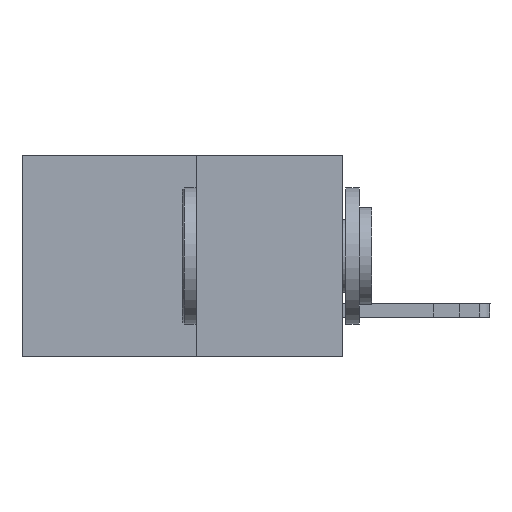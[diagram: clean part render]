
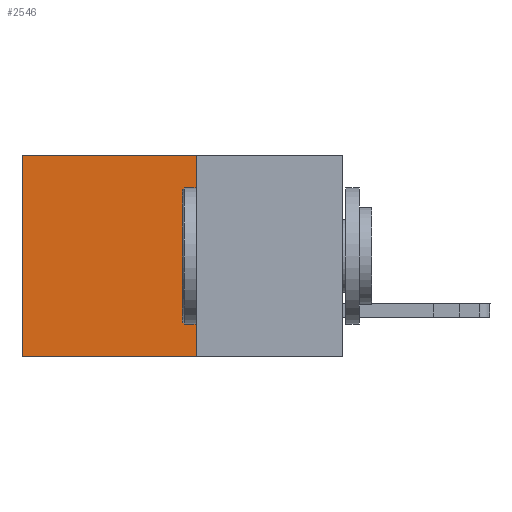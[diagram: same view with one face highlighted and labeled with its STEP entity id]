
A CAD part, left-side view. The second image highlights one B-rep face of the part: STEP entity #2546.
In plain terms, the highlighted planar face has unit normal (-1, 0, 0).
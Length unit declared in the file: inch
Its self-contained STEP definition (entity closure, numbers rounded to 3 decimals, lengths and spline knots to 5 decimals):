
#347 = DIRECTION ( 'NONE',  ( 0., 1., 0. ) ) ;
#481 = CARTESIAN_POINT ( 'NONE',  ( 0.277, 0.27, -0.37 ) ) ;
#568 = EDGE_CURVE ( 'NONE', #18263, #4476, #9971, .T. ) ;
#991 = LINE ( 'NONE', #11039, #9075 ) ;
#2546 = ADVANCED_FACE ( 'NONE', ( #14810 ), #9114, .F. ) ;
#3094 = DIRECTION ( 'NONE',  ( 0., 0., -1. ) ) ;
#3657 = EDGE_CURVE ( 'NONE', #12006, #17336, #9769, .T. ) ;
#4476 = VERTEX_POINT ( 'NONE', #11802 ) ;
#6096 = EDGE_LOOP ( 'NONE', ( #6201, #6909, #7829, #7967 ) ) ;
#6201 = ORIENTED_EDGE ( 'NONE', *, *, #9160, .T. ) ;
#6264 = AXIS2_PLACEMENT_3D ( 'NONE', #7695, #8637, #14380 ) ;
#6376 = LINE ( 'NONE', #13359, #13250 ) ;
#6909 = ORIENTED_EDGE ( 'NONE', *, *, #568, .F. ) ;
#7695 = CARTESIAN_POINT ( 'NONE',  ( 0.277, 0.27, -0.37 ) ) ;
#7829 = ORIENTED_EDGE ( 'NONE', *, *, #8745, .F. ) ;
#7967 = ORIENTED_EDGE ( 'NONE', *, *, #3657, .T. ) ;
#8637 = DIRECTION ( 'NONE',  ( 1., 0., 0. ) ) ;
#8745 = EDGE_CURVE ( 'NONE', #12006, #18263, #6376, .T. ) ;
#9075 = VECTOR ( 'NONE', #3094, 39.37008 ) ;
#9114 = PLANE ( 'NONE',  #6264 ) ;
#9160 = EDGE_CURVE ( 'NONE', #17336, #4476, #991, .T. ) ;
#9166 = CARTESIAN_POINT ( 'NONE',  ( 0.277, 0.27, 0. ) ) ;
#9769 = LINE ( 'NONE', #9166, #17537 ) ;
#9971 = LINE ( 'NONE', #18248, #18209 ) ;
#11039 = CARTESIAN_POINT ( 'NONE',  ( 0.277, 0.59, -0.37 ) ) ;
#11773 = DIRECTION ( 'NONE',  ( 0., 0., -1. ) ) ;
#11802 = CARTESIAN_POINT ( 'NONE',  ( 0.277, 0.59, -0.37 ) ) ;
#12006 = VERTEX_POINT ( 'NONE', #16561 ) ;
#12159 = DIRECTION ( 'NONE',  ( 0., 1., 0. ) ) ;
#13250 = VECTOR ( 'NONE', #11773, 39.37008 ) ;
#13359 = CARTESIAN_POINT ( 'NONE',  ( 0.277, 0.27, -0.37 ) ) ;
#14380 = DIRECTION ( 'NONE',  ( 0., 0., -1. ) ) ;
#14810 = FACE_OUTER_BOUND ( 'NONE', #6096, .T. ) ;
#16561 = CARTESIAN_POINT ( 'NONE',  ( 0.277, 0.27, 0. ) ) ;
#17336 = VERTEX_POINT ( 'NONE', #17423 ) ;
#17423 = CARTESIAN_POINT ( 'NONE',  ( 0.277, 0.59, 0. ) ) ;
#17537 = VECTOR ( 'NONE', #347, 39.37008 ) ;
#18209 = VECTOR ( 'NONE', #12159, 39.37008 ) ;
#18248 = CARTESIAN_POINT ( 'NONE',  ( 0.277, 0.27, -0.37 ) ) ;
#18263 = VERTEX_POINT ( 'NONE', #481 ) ;
